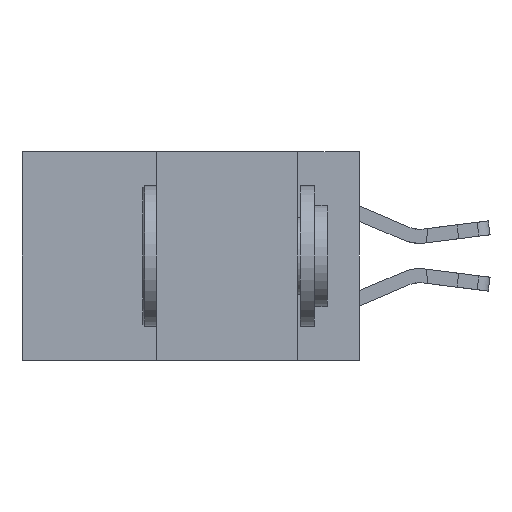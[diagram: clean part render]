
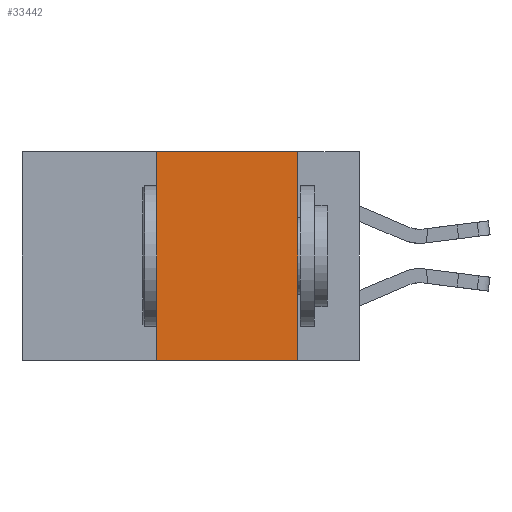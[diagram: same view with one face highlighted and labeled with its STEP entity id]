
A CAD part, left-side view. The second image highlights one B-rep face of the part: STEP entity #33442.
In plain terms, the highlighted planar face has unit normal (-1, 0, 0).
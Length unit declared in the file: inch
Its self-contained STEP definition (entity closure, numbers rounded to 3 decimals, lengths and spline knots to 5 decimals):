
#947 = DIRECTION ( 'NONE',  ( 0., -1., 0. ) ) ;
#1726 = EDGE_LOOP ( 'NONE', ( #9856, #3684, #16961, #23483 ) ) ;
#2338 = PLANE ( 'NONE',  #8648 ) ;
#2399 = LINE ( 'NONE', #26772, #8582 ) ;
#3605 = CARTESIAN_POINT ( 'NONE',  ( 0., 0.36, 0. ) ) ;
#3684 = ORIENTED_EDGE ( 'NONE', *, *, #13271, .F. ) ;
#7890 = CARTESIAN_POINT ( 'NONE',  ( 0., 0.11, 0. ) ) ;
#7991 = CARTESIAN_POINT ( 'NONE',  ( 0., 0.36, 0. ) ) ;
#8169 = CARTESIAN_POINT ( 'NONE',  ( 0., 0.11, 0. ) ) ;
#8582 = VECTOR ( 'NONE', #947, 39.37008 ) ;
#8648 = AXIS2_PLACEMENT_3D ( 'NONE', #12957, #25869, #20890 ) ;
#9856 = ORIENTED_EDGE ( 'NONE', *, *, #23976, .F. ) ;
#10396 = DIRECTION ( 'NONE',  ( 0., 0., -1. ) ) ;
#10426 = LINE ( 'NONE', #7890, #17063 ) ;
#12009 = FACE_OUTER_BOUND ( 'NONE', #1726, .T. ) ;
#12957 = CARTESIAN_POINT ( 'NONE',  ( 0., 0.6, 0. ) ) ;
#13271 = EDGE_CURVE ( 'NONE', #27142, #20995, #2399, .T. ) ;
#16136 = CARTESIAN_POINT ( 'NONE',  ( 0., 0.36, -0.37 ) ) ;
#16796 = EDGE_CURVE ( 'NONE', #23445, #27142, #18587, .T. ) ;
#16961 = ORIENTED_EDGE ( 'NONE', *, *, #16796, .F. ) ;
#17063 = VECTOR ( 'NONE', #10396, 39.37008 ) ;
#18587 = LINE ( 'NONE', #3605, #29706 ) ;
#20890 = DIRECTION ( 'NONE',  ( 0., 0., -1. ) ) ;
#20995 = VERTEX_POINT ( 'NONE', #8169 ) ;
#21775 = CARTESIAN_POINT ( 'NONE',  ( 0., 0.6, -0.37 ) ) ;
#23445 = VERTEX_POINT ( 'NONE', #16136 ) ;
#23483 = ORIENTED_EDGE ( 'NONE', *, *, #32567, .T. ) ;
#23976 = EDGE_CURVE ( 'NONE', #20995, #33648, #10426, .T. ) ;
#24254 = DIRECTION ( 'NONE',  ( 0., 0., 1. ) ) ;
#25869 = DIRECTION ( 'NONE',  ( 1., 0., 0. ) ) ;
#26620 = CARTESIAN_POINT ( 'NONE',  ( 0., 0.11, -0.37 ) ) ;
#26772 = CARTESIAN_POINT ( 'NONE',  ( 0., 0.6, 0. ) ) ;
#27142 = VERTEX_POINT ( 'NONE', #7991 ) ;
#27330 = VECTOR ( 'NONE', #29122, 39.37008 ) ;
#27727 = LINE ( 'NONE', #21775, #27330 ) ;
#29122 = DIRECTION ( 'NONE',  ( 0., -1., 0. ) ) ;
#29706 = VECTOR ( 'NONE', #24254, 39.37008 ) ;
#32567 = EDGE_CURVE ( 'NONE', #23445, #33648, #27727, .T. ) ;
#33442 = ADVANCED_FACE ( 'NONE', ( #12009 ), #2338, .F. ) ;
#33648 = VERTEX_POINT ( 'NONE', #26620 ) ;
